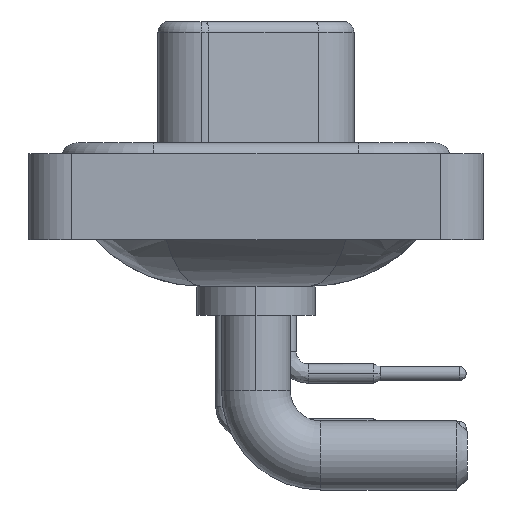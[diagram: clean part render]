
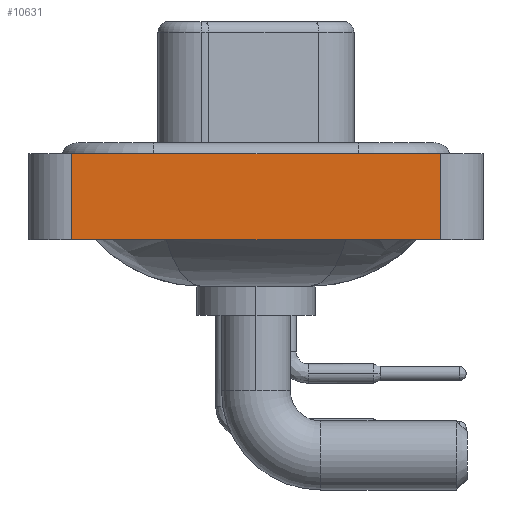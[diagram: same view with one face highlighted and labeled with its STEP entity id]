
A CAD part, left-side view. The second image highlights one B-rep face of the part: STEP entity #10631.
In plain terms, the highlighted planar face has unit normal (-1, 0, 0).
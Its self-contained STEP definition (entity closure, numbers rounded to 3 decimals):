
#547 = CARTESIAN_POINT ( 'NONE',  ( -7.35, -8.55, 0.4 ) ) ;
#2719 = EDGE_LOOP ( 'NONE', ( #17945, #9865, #18680, #23934 ) ) ;
#3198 = LINE ( 'NONE', #26219, #24647 ) ;
#3282 = VECTOR ( 'NONE', #7040, 1000. ) ;
#4147 = VERTEX_POINT ( 'NONE', #23157 ) ;
#4979 = LINE ( 'NONE', #13375, #15167 ) ;
#5034 = EDGE_CURVE ( 'NONE', #7984, #9175, #15457, .T. ) ;
#6511 = LINE ( 'NONE', #12699, #3282 ) ;
#7040 = DIRECTION ( 'NONE',  ( 0., 0., 1. ) ) ;
#7984 = VERTEX_POINT ( 'NONE', #25515 ) ;
#9175 = VERTEX_POINT ( 'NONE', #547 ) ;
#9865 = ORIENTED_EDGE ( 'NONE', *, *, #5034, .F. ) ;
#10631 = ADVANCED_FACE ( 'NONE', ( #18207 ), #24384, .T. ) ;
#12699 = CARTESIAN_POINT ( 'NONE',  ( -7.35, 8.55, -3.6 ) ) ;
#13063 = EDGE_CURVE ( 'NONE', #4147, #7984, #6511, .T. ) ;
#13180 = EDGE_CURVE ( 'NONE', #15206, #9175, #4979, .T. ) ;
#13375 = CARTESIAN_POINT ( 'NONE',  ( -7.35, -8.55, -3.6 ) ) ;
#13508 = CARTESIAN_POINT ( 'NONE',  ( -7.35, -8.55, -3.6 ) ) ;
#14371 = AXIS2_PLACEMENT_3D ( 'NONE', #13508, #16140, #20268 ) ;
#15167 = VECTOR ( 'NONE', #26197, 1000. ) ;
#15206 = VERTEX_POINT ( 'NONE', #15941 ) ;
#15457 = LINE ( 'NONE', #17123, #20363 ) ;
#15941 = CARTESIAN_POINT ( 'NONE',  ( -7.35, -8.55, -3.6 ) ) ;
#16140 = DIRECTION ( 'NONE',  ( -1., 0., 0. ) ) ;
#17123 = CARTESIAN_POINT ( 'NONE',  ( -7.35, -8.55, 0.4 ) ) ;
#17397 = DIRECTION ( 'NONE',  ( 0., -1., 0. ) ) ;
#17945 = ORIENTED_EDGE ( 'NONE', *, *, #13180, .T. ) ;
#18207 = FACE_OUTER_BOUND ( 'NONE', #2719, .T. ) ;
#18680 = ORIENTED_EDGE ( 'NONE', *, *, #13063, .F. ) ;
#20268 = DIRECTION ( 'NONE',  ( 0., 0., 1. ) ) ;
#20363 = VECTOR ( 'NONE', #17397, 1000. ) ;
#23157 = CARTESIAN_POINT ( 'NONE',  ( -7.35, 8.55, -3.6 ) ) ;
#23934 = ORIENTED_EDGE ( 'NONE', *, *, #26096, .T. ) ;
#24384 = PLANE ( 'NONE',  #14371 ) ;
#24647 = VECTOR ( 'NONE', #26771, 1000. ) ;
#25515 = CARTESIAN_POINT ( 'NONE',  ( -7.35, 8.55, 0.4 ) ) ;
#26096 = EDGE_CURVE ( 'NONE', #4147, #15206, #3198, .T. ) ;
#26197 = DIRECTION ( 'NONE',  ( 0., 0., 1. ) ) ;
#26219 = CARTESIAN_POINT ( 'NONE',  ( -7.35, -8.55, -3.6 ) ) ;
#26771 = DIRECTION ( 'NONE',  ( 0., -1., 0. ) ) ;
